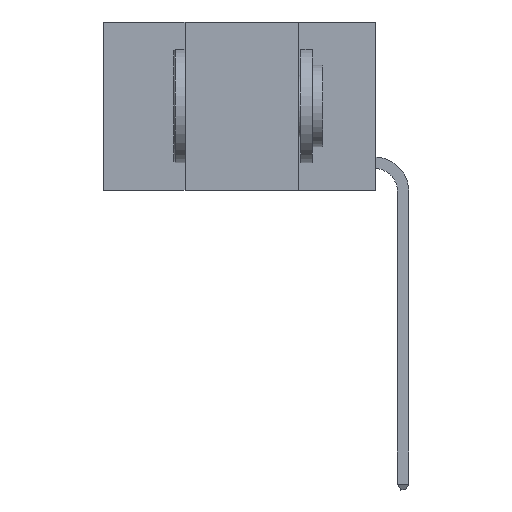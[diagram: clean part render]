
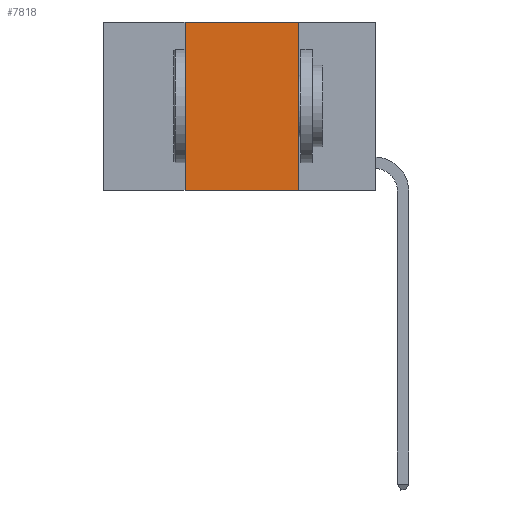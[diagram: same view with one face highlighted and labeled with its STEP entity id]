
A CAD part, left-side view. The second image highlights one B-rep face of the part: STEP entity #7818.
In plain terms, the highlighted planar face has unit normal (-1, 0, 0).
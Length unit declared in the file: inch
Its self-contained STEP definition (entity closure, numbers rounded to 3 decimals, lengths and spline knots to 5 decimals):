
#215 = VECTOR ( 'NONE', #5995, 39.37008 ) ;
#575 = ORIENTED_EDGE ( 'NONE', *, *, #6815, .F. ) ;
#594 = CARTESIAN_POINT ( 'NONE',  ( 0., 0.42, 0. ) ) ;
#633 = CARTESIAN_POINT ( 'NONE',  ( 0., 0.17, 0. ) ) ;
#1229 = VERTEX_POINT ( 'NONE', #594 ) ;
#1291 = CARTESIAN_POINT ( 'NONE',  ( 0., 0.6, 0. ) ) ;
#1776 = CARTESIAN_POINT ( 'NONE',  ( 0., 0.42, -0.37 ) ) ;
#2123 = CARTESIAN_POINT ( 'NONE',  ( 0., 0.42, 0. ) ) ;
#2343 = CARTESIAN_POINT ( 'NONE',  ( 0., 0.17, 0. ) ) ;
#2804 = LINE ( 'NONE', #2123, #4143 ) ;
#2889 = CARTESIAN_POINT ( 'NONE',  ( 0., 0.6, -0.37 ) ) ;
#2912 = DIRECTION ( 'NONE',  ( 0., -1., 0. ) ) ;
#2942 = DIRECTION ( 'NONE',  ( 0., 0., 1. ) ) ;
#4143 = VECTOR ( 'NONE', #2942, 39.37008 ) ;
#4822 = VECTOR ( 'NONE', #7519, 39.37008 ) ;
#4938 = DIRECTION ( 'NONE',  ( 0., 0., -1. ) ) ;
#5338 = VECTOR ( 'NONE', #2912, 39.37008 ) ;
#5466 = EDGE_CURVE ( 'NONE', #1229, #9142, #6625, .T. ) ;
#5856 = VERTEX_POINT ( 'NONE', #1776 ) ;
#5995 = DIRECTION ( 'NONE',  ( 0., 0., -1. ) ) ;
#6552 = VERTEX_POINT ( 'NONE', #7268 ) ;
#6625 = LINE ( 'NONE', #1291, #5338 ) ;
#6654 = ORIENTED_EDGE ( 'NONE', *, *, #8564, .T. ) ;
#6815 = EDGE_CURVE ( 'NONE', #9142, #6552, #7456, .T. ) ;
#7167 = DIRECTION ( 'NONE',  ( 1., 0., 0. ) ) ;
#7196 = ORIENTED_EDGE ( 'NONE', *, *, #9876, .F. ) ;
#7268 = CARTESIAN_POINT ( 'NONE',  ( 0., 0.17, -0.37 ) ) ;
#7456 = LINE ( 'NONE', #633, #215 ) ;
#7519 = DIRECTION ( 'NONE',  ( 0., -1., 0. ) ) ;
#7818 = ADVANCED_FACE ( 'NONE', ( #8028 ), #9486, .F. ) ;
#8028 = FACE_OUTER_BOUND ( 'NONE', #8577, .T. ) ;
#8564 = EDGE_CURVE ( 'NONE', #5856, #6552, #9048, .T. ) ;
#8577 = EDGE_LOOP ( 'NONE', ( #575, #8702, #7196, #6654 ) ) ;
#8702 = ORIENTED_EDGE ( 'NONE', *, *, #5466, .F. ) ;
#8849 = CARTESIAN_POINT ( 'NONE',  ( 0., 0.6, 0. ) ) ;
#9048 = LINE ( 'NONE', #2889, #4822 ) ;
#9142 = VERTEX_POINT ( 'NONE', #2343 ) ;
#9422 = AXIS2_PLACEMENT_3D ( 'NONE', #8849, #7167, #4938 ) ;
#9486 = PLANE ( 'NONE',  #9422 ) ;
#9876 = EDGE_CURVE ( 'NONE', #5856, #1229, #2804, .T. ) ;
